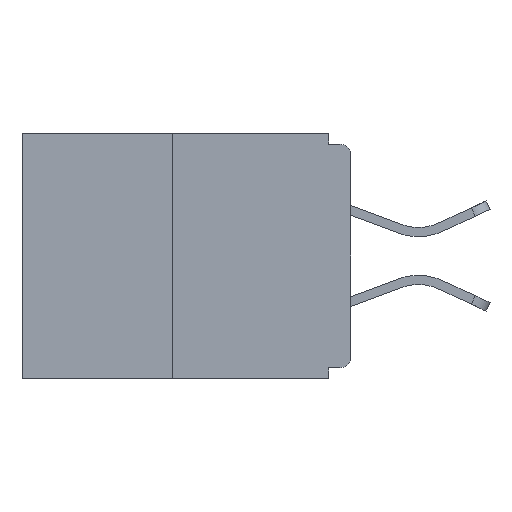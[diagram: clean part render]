
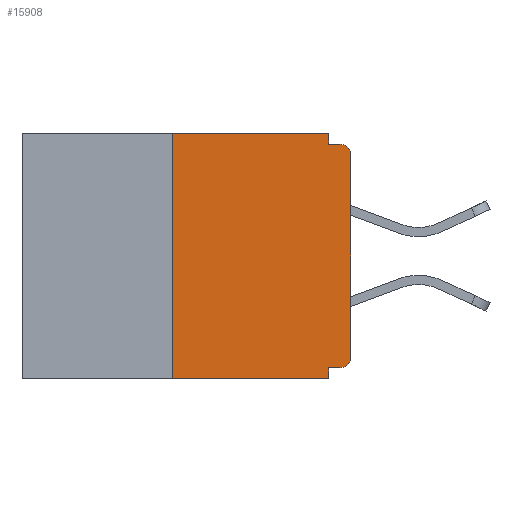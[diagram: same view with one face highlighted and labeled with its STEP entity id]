
A CAD part, left-side view. The second image highlights one B-rep face of the part: STEP entity #15908.
In plain terms, the highlighted planar face has unit normal (-1, 0, 0).
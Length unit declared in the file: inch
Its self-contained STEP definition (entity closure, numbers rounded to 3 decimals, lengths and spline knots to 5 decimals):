
#833 = VERTEX_POINT ( 'NONE', #10916 ) ;
#1261 = EDGE_CURVE ( 'NONE', #833, #16726, #19119, .T. ) ;
#1807 = CARTESIAN_POINT ( 'NONE',  ( 0., 0., -0.03 ) ) ;
#2427 = EDGE_CURVE ( 'NONE', #4394, #9032, #8413, .T. ) ;
#2436 = VECTOR ( 'NONE', #14149, 39.37008 ) ;
#2735 = CARTESIAN_POINT ( 'NONE',  ( 0., 0.031, 0. ) ) ;
#2971 = CARTESIAN_POINT ( 'NONE',  ( 0., 0.25, -0.343 ) ) ;
#3219 = DIRECTION ( 'NONE',  ( 0., 0., -1. ) ) ;
#3475 = LINE ( 'NONE', #4491, #21375 ) ;
#3533 = CARTESIAN_POINT ( 'NONE',  ( 0., 0.25, 0. ) ) ;
#3728 = EDGE_CURVE ( 'NONE', #9088, #21900, #4281, .T. ) ;
#3820 = AXIS2_PLACEMENT_3D ( 'NONE', #22529, #8325, #22372 ) ;
#4251 = CARTESIAN_POINT ( 'NONE',  ( 0., 0.015, -0.328 ) ) ;
#4281 = CIRCLE ( 'NONE', #6653, 0.015 ) ;
#4394 = VERTEX_POINT ( 'NONE', #1807 ) ;
#4491 = CARTESIAN_POINT ( 'NONE',  ( 0., 0., -0.328 ) ) ;
#4988 = DIRECTION ( 'NONE',  ( 0., -1., 0. ) ) ;
#5038 = ORIENTED_EDGE ( 'NONE', *, *, #3728, .T. ) ;
#5105 = CARTESIAN_POINT ( 'NONE',  ( 0., 0.031, -0.328 ) ) ;
#5511 = ORIENTED_EDGE ( 'NONE', *, *, #20074, .F. ) ;
#6122 = VECTOR ( 'NONE', #4988, 39.37008 ) ;
#6256 = DIRECTION ( 'NONE',  ( 0., -1., 0. ) ) ;
#6371 = EDGE_CURVE ( 'NONE', #7686, #9943, #10217, .T. ) ;
#6576 = EDGE_CURVE ( 'NONE', #9616, #9943, #22841, .T. ) ;
#6653 = AXIS2_PLACEMENT_3D ( 'NONE', #13103, #14905, #9729 ) ;
#6859 = CARTESIAN_POINT ( 'NONE',  ( 0., 0., -0.015 ) ) ;
#6900 = FACE_OUTER_BOUND ( 'NONE', #8417, .T. ) ;
#6997 = DIRECTION ( 'NONE',  ( 0., 0., 1. ) ) ;
#7391 = ORIENTED_EDGE ( 'NONE', *, *, #14701, .T. ) ;
#7686 = VERTEX_POINT ( 'NONE', #2971 ) ;
#7780 = CARTESIAN_POINT ( 'NONE',  ( 0., 0.031, -0.015 ) ) ;
#7793 = LINE ( 'NONE', #6859, #6122 ) ;
#8083 = DIRECTION ( 'NONE',  ( 0., 0., -1. ) ) ;
#8325 = DIRECTION ( 'NONE',  ( -1., 0., 0. ) ) ;
#8342 = EDGE_CURVE ( 'NONE', #9088, #9616, #3475, .T. ) ;
#8413 = CIRCLE ( 'NONE', #3820, 0.015 ) ;
#8417 = EDGE_LOOP ( 'NONE', ( #15990, #20512, #19231, #22388, #19252, #5038, #7391, #9803, #5511, #11956 ) ) ;
#9032 = VERTEX_POINT ( 'NONE', #18423 ) ;
#9087 = DIRECTION ( 'NONE',  ( 0., -1., 0. ) ) ;
#9088 = VERTEX_POINT ( 'NONE', #4251 ) ;
#9616 = VERTEX_POINT ( 'NONE', #5105 ) ;
#9729 = DIRECTION ( 'NONE',  ( 0., 0., -1. ) ) ;
#9803 = ORIENTED_EDGE ( 'NONE', *, *, #2427, .T. ) ;
#9943 = VERTEX_POINT ( 'NONE', #16979 ) ;
#10217 = LINE ( 'NONE', #11689, #15411 ) ;
#10916 = CARTESIAN_POINT ( 'NONE',  ( 0., 0.031, 0. ) ) ;
#11689 = CARTESIAN_POINT ( 'NONE',  ( 0., 0.46, -0.343 ) ) ;
#11706 = DIRECTION ( 'NONE',  ( 0., 1., 0. ) ) ;
#11852 = CARTESIAN_POINT ( 'NONE',  ( 0., 0., 0. ) ) ;
#11956 = ORIENTED_EDGE ( 'NONE', *, *, #1261, .F. ) ;
#12409 = LINE ( 'NONE', #11852, #21554 ) ;
#12507 = EDGE_CURVE ( 'NONE', #7686, #13073, #21063, .T. ) ;
#12875 = CARTESIAN_POINT ( 'NONE',  ( 0., 0.25, 0. ) ) ;
#13073 = VERTEX_POINT ( 'NONE', #12875 ) ;
#13103 = CARTESIAN_POINT ( 'NONE',  ( 0., 0.015, -0.313 ) ) ;
#13631 = CARTESIAN_POINT ( 'NONE',  ( 0., 0.46, 0. ) ) ;
#14028 = VECTOR ( 'NONE', #9087, 39.37008 ) ;
#14071 = CARTESIAN_POINT ( 'NONE',  ( 0., 0.031, -0.343 ) ) ;
#14149 = DIRECTION ( 'NONE',  ( 0., 0., -1. ) ) ;
#14259 = CARTESIAN_POINT ( 'NONE',  ( 0., 0.46, 0. ) ) ;
#14701 = EDGE_CURVE ( 'NONE', #21900, #4394, #12409, .T. ) ;
#14905 = DIRECTION ( 'NONE',  ( -1., 0., 0. ) ) ;
#15411 = VECTOR ( 'NONE', #6256, 39.37008 ) ;
#15430 = DIRECTION ( 'NONE',  ( 1., 0., 0. ) ) ;
#15908 = ADVANCED_FACE ( 'NONE', ( #6900 ), #22448, .F. ) ;
#15990 = ORIENTED_EDGE ( 'NONE', *, *, #16047, .F. ) ;
#16047 = EDGE_CURVE ( 'NONE', #13073, #833, #17068, .T. ) ;
#16123 = VECTOR ( 'NONE', #6997, 39.37008 ) ;
#16499 = AXIS2_PLACEMENT_3D ( 'NONE', #13631, #15430, #3219 ) ;
#16726 = VERTEX_POINT ( 'NONE', #7780 ) ;
#16979 = CARTESIAN_POINT ( 'NONE',  ( 0., 0.031, -0.343 ) ) ;
#17068 = LINE ( 'NONE', #14259, #14028 ) ;
#18032 = VECTOR ( 'NONE', #8083, 39.37008 ) ;
#18423 = CARTESIAN_POINT ( 'NONE',  ( 0., 0.015, -0.015 ) ) ;
#19119 = LINE ( 'NONE', #2735, #18032 ) ;
#19231 = ORIENTED_EDGE ( 'NONE', *, *, #6371, .T. ) ;
#19252 = ORIENTED_EDGE ( 'NONE', *, *, #8342, .F. ) ;
#20074 = EDGE_CURVE ( 'NONE', #16726, #9032, #7793, .T. ) ;
#20512 = ORIENTED_EDGE ( 'NONE', *, *, #12507, .F. ) ;
#20636 = DIRECTION ( 'NONE',  ( 0., 0., 1. ) ) ;
#21063 = LINE ( 'NONE', #3533, #16123 ) ;
#21375 = VECTOR ( 'NONE', #11706, 39.37008 ) ;
#21554 = VECTOR ( 'NONE', #20636, 39.37008 ) ;
#21900 = VERTEX_POINT ( 'NONE', #22228 ) ;
#22228 = CARTESIAN_POINT ( 'NONE',  ( 0., 0., -0.313 ) ) ;
#22372 = DIRECTION ( 'NONE',  ( 0., 0., -1. ) ) ;
#22388 = ORIENTED_EDGE ( 'NONE', *, *, #6576, .F. ) ;
#22448 = PLANE ( 'NONE',  #16499 ) ;
#22529 = CARTESIAN_POINT ( 'NONE',  ( 0., 0.015, -0.03 ) ) ;
#22841 = LINE ( 'NONE', #14071, #2436 ) ;
